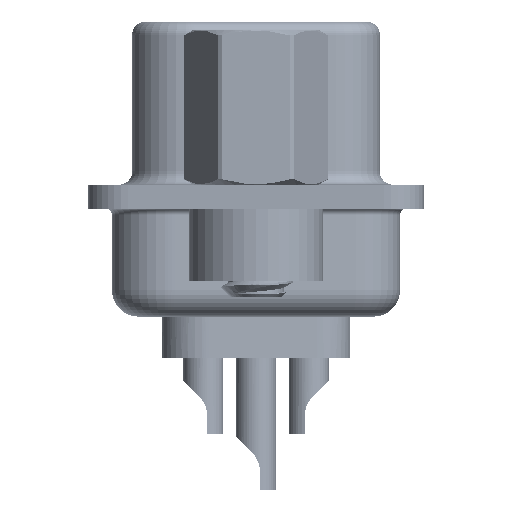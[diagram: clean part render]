
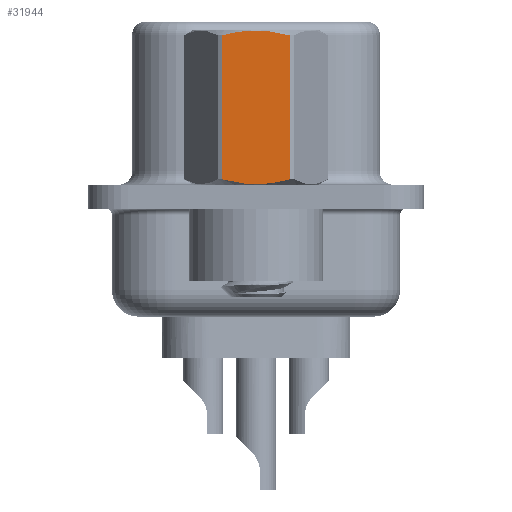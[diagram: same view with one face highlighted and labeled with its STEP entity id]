
A CAD part, left-side view. The second image highlights one B-rep face of the part: STEP entity #31944.
In plain terms, the highlighted planar face has unit normal (-1, 0, 0).
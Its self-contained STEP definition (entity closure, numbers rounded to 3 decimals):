
#1176 = CARTESIAN_POINT ( 'NONE',  ( -2.381, 0.215, 0.468 ) ) ;
#1404 = CARTESIAN_POINT ( 'NONE',  ( -2.381, 0.215, 6.232 ) ) ;
#1683 = CARTESIAN_POINT ( 'NONE',  ( -2.381, 1.065, 0.596 ) ) ;
#2047 = ORIENTED_EDGE ( 'NONE', *, *, #29668, .T. ) ;
#2511 = EDGE_CURVE ( 'NONE', #24223, #8503, #26926, .T. ) ;
#3026 = DIRECTION ( 'NONE',  ( 0., 0., 1. ) ) ;
#3947 = CARTESIAN_POINT ( 'NONE',  ( -2.381, 0.428, 0.485 ) ) ;
#3994 = CARTESIAN_POINT ( 'NONE',  ( -2.381, 1.375, -3.75 ) ) ;
#4846 = DIRECTION ( 'NONE',  ( 0., 0., -1. ) ) ;
#5054 = VECTOR ( 'NONE', #3026, 1000. ) ;
#6748 = CARTESIAN_POINT ( 'NONE',  ( -2.381, -0.215, 0.468 ) ) ;
#6799 = FACE_OUTER_BOUND ( 'NONE', #26597, .T. ) ;
#7154 = CARTESIAN_POINT ( 'NONE',  ( -2.381, 0.853, 6.151 ) ) ;
#7593 = EDGE_CURVE ( 'NONE', #8503, #26979, #11194, .T. ) ;
#7623 = CARTESIAN_POINT ( 'NONE',  ( -2.381, 1.273, 0.652 ) ) ;
#8503 = VERTEX_POINT ( 'NONE', #27809 ) ;
#9705 = CARTESIAN_POINT ( 'NONE',  ( -2.381, -0.858, 0.55 ) ) ;
#9766 = CARTESIAN_POINT ( 'NONE',  ( -2.381, -0.858, 6.15 ) ) ;
#11194 = B_SPLINE_CURVE_WITH_KNOTS ( 'NONE', 3,
 ( #25289, #11892, #9766, #30974, #14987, #1404, #12059, #7154, #22672, #33252 ),
 .UNSPECIFIED., .F., .F.,
 ( 4, 2, 2, 2, 4 ),
 ( 0.001, 0.002, 0.002, 0.003, 0.004 ),
 .UNSPECIFIED. ) ;
#11198 = B_SPLINE_CURVE_WITH_KNOTS ( 'NONE', 3,
 ( #25571, #1683, #12332, #3947, #1176, #6748, #17045, #9705, #19652, #25399 ),
 .UNSPECIFIED., .F., .F.,
 ( 4, 2, 2, 2, 4 ),
 ( 0.003, 0.003, 0.004, 0.004, 0.005 ),
 .UNSPECIFIED. ) ;
#11249 = ORIENTED_EDGE ( 'NONE', *, *, #2511, .T. ) ;
#11892 = CARTESIAN_POINT ( 'NONE',  ( -2.381, -1.066, 6.104 ) ) ;
#12059 = CARTESIAN_POINT ( 'NONE',  ( -2.381, 0.428, 6.215 ) ) ;
#12332 = CARTESIAN_POINT ( 'NONE',  ( -2.381, 0.853, 0.549 ) ) ;
#14987 = CARTESIAN_POINT ( 'NONE',  ( -2.381, -0.215, 6.232 ) ) ;
#15296 = CARTESIAN_POINT ( 'NONE',  ( -2.381, -1.273, 3.792 ) ) ;
#17045 = CARTESIAN_POINT ( 'NONE',  ( -2.381, -0.432, 0.485 ) ) ;
#17601 = AXIS2_PLACEMENT_3D ( 'NONE', #3994, #20380, #28565 ) ;
#17766 = CARTESIAN_POINT ( 'NONE',  ( -2.381, -1.273, 0.652 ) ) ;
#19652 = CARTESIAN_POINT ( 'NONE',  ( -2.381, -1.066, 0.596 ) ) ;
#20380 = DIRECTION ( 'NONE',  ( -1., 0., 0. ) ) ;
#22672 = CARTESIAN_POINT ( 'NONE',  ( -2.381, 1.065, 6.104 ) ) ;
#22833 = PLANE ( 'NONE',  #17601 ) ;
#24223 = VERTEX_POINT ( 'NONE', #17766 ) ;
#25289 = CARTESIAN_POINT ( 'NONE',  ( -2.381, -1.273, 6.048 ) ) ;
#25399 = CARTESIAN_POINT ( 'NONE',  ( -2.381, -1.273, 0.652 ) ) ;
#25571 = CARTESIAN_POINT ( 'NONE',  ( -2.381, 1.273, 0.652 ) ) ;
#25614 = ORIENTED_EDGE ( 'NONE', *, *, #29812, .T. ) ;
#25826 = VECTOR ( 'NONE', #4846, 1000. ) ;
#26597 = EDGE_LOOP ( 'NONE', ( #25614, #11249, #27576, #2047 ) ) ;
#26926 = LINE ( 'NONE', #15296, #5054 ) ;
#26979 = VERTEX_POINT ( 'NONE', #32593 ) ;
#27576 = ORIENTED_EDGE ( 'NONE', *, *, #7593, .T. ) ;
#27809 = CARTESIAN_POINT ( 'NONE',  ( -2.381, -1.273, 6.048 ) ) ;
#28565 = DIRECTION ( 'NONE',  ( 0., -1., 0. ) ) ;
#29668 = EDGE_CURVE ( 'NONE', #26979, #30733, #31641, .T. ) ;
#29812 = EDGE_CURVE ( 'NONE', #30733, #24223, #11198, .T. ) ;
#30733 = VERTEX_POINT ( 'NONE', #7623 ) ;
#30974 = CARTESIAN_POINT ( 'NONE',  ( -2.381, -0.432, 6.215 ) ) ;
#31641 = LINE ( 'NONE', #33916, #25826 ) ;
#31944 = ADVANCED_FACE ( 'NONE', ( #6799 ), #22833, .T. ) ;
#32593 = CARTESIAN_POINT ( 'NONE',  ( -2.381, 1.273, 6.048 ) ) ;
#33252 = CARTESIAN_POINT ( 'NONE',  ( -2.381, 1.273, 6.048 ) ) ;
#33916 = CARTESIAN_POINT ( 'NONE',  ( -2.381, 1.273, 3.792 ) ) ;
